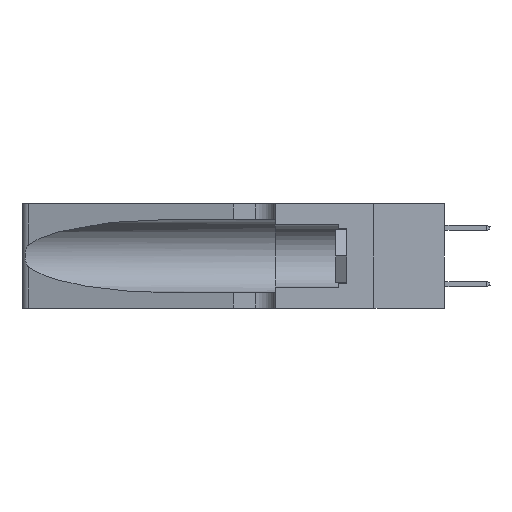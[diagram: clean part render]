
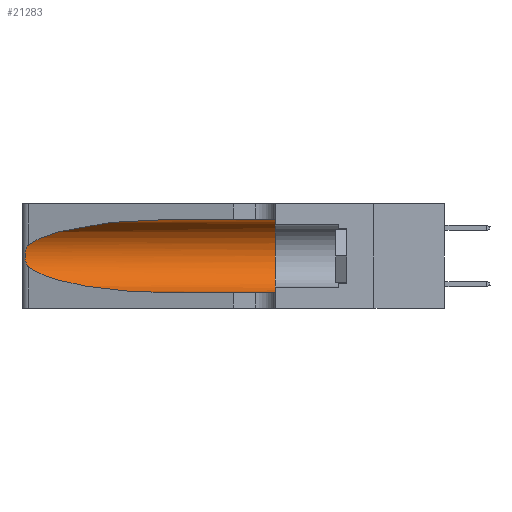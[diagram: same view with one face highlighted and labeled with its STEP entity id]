
A CAD part, left-side view. The second image highlights one B-rep face of the part: STEP entity #21283.
In plain terms, the highlighted cylindrical face has radius 3.308 mm (diameter 6.617 mm), a partial arc.
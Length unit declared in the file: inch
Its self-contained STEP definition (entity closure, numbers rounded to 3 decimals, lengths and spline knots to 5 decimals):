
#120 = CARTESIAN_POINT ( 'NONE',  ( 0.26075, 1.23896, 0.19203 ) ) ;
#343 = B_SPLINE_CURVE_WITH_KNOTS ( 'NONE', 3,
 ( #9564, #28232, #34409, #15886, #37540, #18996, #120, #22122, #3318, #25256, #6531, #28359, #9696, #31454 ),
 .UNSPECIFIED., .F., .F.,
 ( 4, 2, 2, 2, 2, 2, 4 ),
 ( 0., 0.00027, 0.00053, 0.00107, 0.0016, 0.00187, 0.00214 ),
 .UNSPECIFIED. ) ;
#901 = VERTEX_POINT ( 'NONE', #31923 ) ;
#1208 = VERTEX_POINT ( 'NONE', #8369 ) ;
#1423 = CARTESIAN_POINT ( 'NONE',  ( 0.25487, 1.22718, 0.22369 ) ) ;
#1972 = CARTESIAN_POINT ( 'NONE',  ( 0.25487, 1.22718, 0.22369 ) ) ;
#2603 = ORIENTED_EDGE ( 'NONE', *, *, #32688, .T. ) ;
#3073 = CARTESIAN_POINT ( 'NONE',  ( 0.1305, 0.72297, 0.31525 ) ) ;
#3318 = CARTESIAN_POINT ( 'NONE',  ( 0.26017, 1.23833, 0.17102 ) ) ;
#3733 = CARTESIAN_POINT ( 'NONE',  ( 0.1305, 0.35, 0.185 ) ) ;
#4239 = VERTEX_POINT ( 'NONE', #1423 ) ;
#6531 = CARTESIAN_POINT ( 'NONE',  ( 0.25789, 1.23486, 0.15765 ) ) ;
#6936 = DIRECTION ( 'NONE',  ( 0., 0., 1. ) ) ;
#7523 = AXIS2_PLACEMENT_3D ( 'NONE', #21513, #18267, #12152 ) ;
#7696 = ORIENTED_EDGE ( 'NONE', *, *, #32503, .T. ) ;
#7752 =( BOUNDED_CURVE ( )  B_SPLINE_CURVE ( 3, ( #29845, #8073, #17507, #39145 ),
 .UNSPECIFIED., .F., .T. ) 
 B_SPLINE_CURVE_WITH_KNOTS ( ( 4, 4 ),
 ( 3.44316, 4.71239 ),
 .UNSPECIFIED. ) 
 CURVE ( )  GEOMETRIC_REPRESENTATION_ITEM ( )  RATIONAL_B_SPLINE_CURVE ( ( 1., 0.87, 0.87, 1. ) ) 
 REPRESENTATION_ITEM ( '' )  );
#8073 = CARTESIAN_POINT ( 'NONE',  ( 0.2373, 1.15595, 0.08982 ) ) ;
#8369 = CARTESIAN_POINT ( 'NONE',  ( 0.1305, 0.35, 0.31525 ) ) ;
#8565 = LINE ( 'NONE', #23846, #24205 ) ;
#9464 = VECTOR ( 'NONE', #14420, 39.37008 ) ;
#9564 = CARTESIAN_POINT ( 'NONE',  ( 0.25487, 1.22718, 0.22369 ) ) ;
#9696 = CARTESIAN_POINT ( 'NONE',  ( 0.25555, 1.22993, 0.14849 ) ) ;
#10446 = ORIENTED_EDGE ( 'NONE', *, *, #22546, .T. ) ;
#11256 = CARTESIAN_POINT ( 'NONE',  ( 0.1305, 1.61858, 0.31525 ) ) ;
#12152 = DIRECTION ( 'NONE',  ( 0., 0., -1. ) ) ;
#12943 = VERTEX_POINT ( 'NONE', #20504 ) ;
#13979 = CIRCLE ( 'NONE', #17663, 0.13025 ) ;
#14420 = DIRECTION ( 'NONE',  ( 0., -1., 0. ) ) ;
#15683 = EDGE_CURVE ( 'NONE', #12943, #25200, #8565, .T. ) ;
#15886 = CARTESIAN_POINT ( 'NONE',  ( 0.25787, 1.23484, 0.2124 ) ) ;
#16963 = EDGE_CURVE ( 'NONE', #1208, #25200, #13979, .T. ) ;
#17507 = CARTESIAN_POINT ( 'NONE',  ( 0.18966, 0.96281, 0.05475 ) ) ;
#17663 = AXIS2_PLACEMENT_3D ( 'NONE', #3733, #25629, #6936 ) ;
#18267 = DIRECTION ( 'NONE',  ( 0., -1., 0. ) ) ;
#18996 = CARTESIAN_POINT ( 'NONE',  ( 0.26018, 1.23835, 0.19895 ) ) ;
#20504 = CARTESIAN_POINT ( 'NONE',  ( 0.1305, 0.72297, 0.05475 ) ) ;
#20820 = CARTESIAN_POINT ( 'NONE',  ( 0.2373, 1.15595, 0.28018 ) ) ;
#21283 = ADVANCED_FACE ( 'NONE', ( #33780 ), #32821, .F. ) ;
#21513 = CARTESIAN_POINT ( 'NONE',  ( 0.1305, 1.61858, 0.185 ) ) ;
#22122 = CARTESIAN_POINT ( 'NONE',  ( 0.26075, 1.23896, 0.178 ) ) ;
#22546 = EDGE_CURVE ( 'NONE', #32162, #4239, #29476, .T. ) ;
#23846 = CARTESIAN_POINT ( 'NONE',  ( 0.1305, 1.61858, 0.05475 ) ) ;
#24205 = VECTOR ( 'NONE', #30056, 39.37008 ) ;
#25200 = VERTEX_POINT ( 'NONE', #36286 ) ;
#25256 = CARTESIAN_POINT ( 'NONE',  ( 0.25856, 1.23593, 0.16098 ) ) ;
#25629 = DIRECTION ( 'NONE',  ( 0., 1., 0. ) ) ;
#26730 = ORIENTED_EDGE ( 'NONE', *, *, #16963, .F. ) ;
#28232 = CARTESIAN_POINT ( 'NONE',  ( 0.25555, 1.22994, 0.2215 ) ) ;
#28359 = CARTESIAN_POINT ( 'NONE',  ( 0.25639, 1.23186, 0.15144 ) ) ;
#29476 =( BOUNDED_CURVE ( )  B_SPLINE_CURVE ( 3, ( #30026, #33109, #20820, #1972 ),
 .UNSPECIFIED., .F., .F. ) 
 B_SPLINE_CURVE_WITH_KNOTS ( ( 4, 4 ),
 ( 1.5708, 2.84003 ),
 .UNSPECIFIED. ) 
 CURVE ( )  GEOMETRIC_REPRESENTATION_ITEM ( )  RATIONAL_B_SPLINE_CURVE ( ( 1., 0.87, 0.87, 1. ) ) 
 REPRESENTATION_ITEM ( '' )  );
#29845 = CARTESIAN_POINT ( 'NONE',  ( 0.25487, 1.22718, 0.14631 ) ) ;
#30026 = CARTESIAN_POINT ( 'NONE',  ( 0.1305, 0.72297, 0.31525 ) ) ;
#30056 = DIRECTION ( 'NONE',  ( 0., -1., 0. ) ) ;
#31454 = CARTESIAN_POINT ( 'NONE',  ( 0.25487, 1.22718, 0.14631 ) ) ;
#31923 = CARTESIAN_POINT ( 'NONE',  ( 0.25487, 1.22718, 0.14631 ) ) ;
#32162 = VERTEX_POINT ( 'NONE', #3073 ) ;
#32503 = EDGE_CURVE ( 'NONE', #901, #12943, #7752, .T. ) ;
#32688 = EDGE_CURVE ( 'NONE', #4239, #901, #343, .T. ) ;
#32802 = EDGE_LOOP ( 'NONE', ( #10446, #2603, #7696, #36810, #26730, #35775 ) ) ;
#32821 = CYLINDRICAL_SURFACE ( 'NONE', #7523, 0.13025 ) ;
#33109 = CARTESIAN_POINT ( 'NONE',  ( 0.18966, 0.96281, 0.31525 ) ) ;
#33280 = LINE ( 'NONE', #11256, #9464 ) ;
#33780 = FACE_OUTER_BOUND ( 'NONE', #32802, .T. ) ;
#34409 = CARTESIAN_POINT ( 'NONE',  ( 0.25639, 1.23184, 0.21858 ) ) ;
#35775 = ORIENTED_EDGE ( 'NONE', *, *, #38878, .F. ) ;
#36286 = CARTESIAN_POINT ( 'NONE',  ( 0.1305, 0.35, 0.05475 ) ) ;
#36810 = ORIENTED_EDGE ( 'NONE', *, *, #15683, .T. ) ;
#37540 = CARTESIAN_POINT ( 'NONE',  ( 0.25854, 1.2359, 0.20912 ) ) ;
#38878 = EDGE_CURVE ( 'NONE', #32162, #1208, #33280, .T. ) ;
#39145 = CARTESIAN_POINT ( 'NONE',  ( 0.1305, 0.72297, 0.05475 ) ) ;
